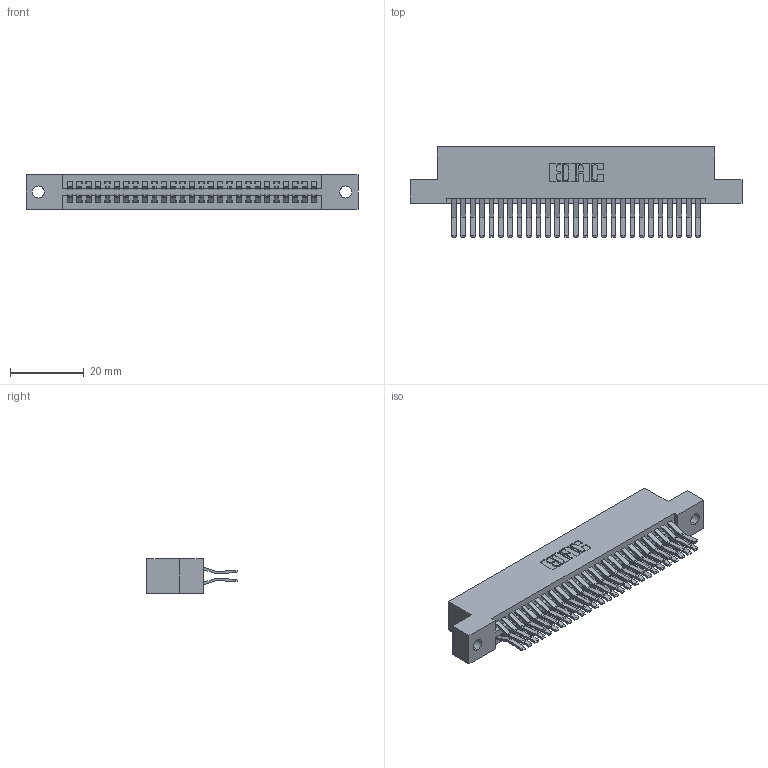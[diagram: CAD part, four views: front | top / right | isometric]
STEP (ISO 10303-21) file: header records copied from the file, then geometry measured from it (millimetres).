
FILE_DESCRIPTION (( 'STEP AP203' ), '1' );
FILE_NAME ('395-054-560-202.STEP', '2019-10-19T17:51:48', ( '' ), ( '' ), 'SwSTEP 2.0', 'SolidWorks 2016', '' );
FILE_SCHEMA (( 'CONFIG_CONTROL_DESIGN' ));
Length unit declared in the file: inch
Products named in the file (3): 345 Part_Flush Mounting Lugs - 0.128 Dia; 345-292-001_560 Tail; 395-054-560-202
Assembly tree (55 placements, depth 2):
  395-054-560-202
    345 Part_Flush Mounting Lugs - 0.128 Dia
    345-292-001_560 Tail  x54
Bounding box: 89.79 x 24.45 x 9.4 mm (x, y, z)
Volume: 8900.2 mm3; surface area: 13503.1 mm2
Topology: 55 solids, 55 shells, 2934 faces, 8711 edges, 5734 vertices
Faces by surface type: plane 1862, cylinder 1072
Entity records: 23295 total; most frequent: CARTESIAN_POINT 3920, ORIENTED_EDGE 3854, DIRECTION 3479, EDGE_CURVE 1927, LINE 1683, VECTOR 1683, VERTEX_POINT 1282, AXIS2_PLACEMENT_3D 898
